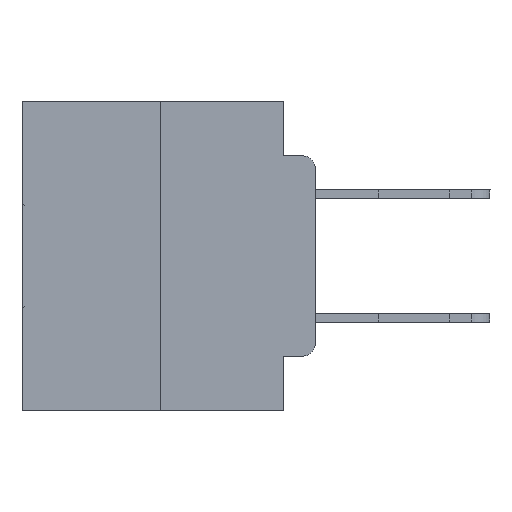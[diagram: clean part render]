
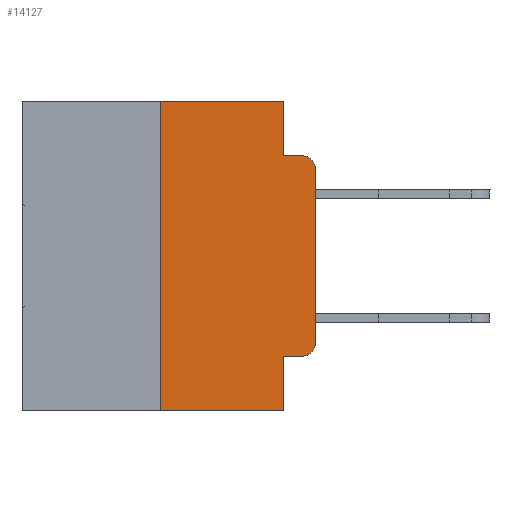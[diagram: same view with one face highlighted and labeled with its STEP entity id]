
A CAD part, left-side view. The second image highlights one B-rep face of the part: STEP entity #14127.
In plain terms, the highlighted planar face has unit normal (-1, 0, 0).
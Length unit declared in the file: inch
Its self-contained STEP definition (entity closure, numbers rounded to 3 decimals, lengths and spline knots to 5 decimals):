
#339 = VERTEX_POINT ( 'NONE', #20694 ) ;
#368 = FACE_OUTER_BOUND ( 'NONE', #4620, .T. ) ;
#550 = EDGE_CURVE ( 'NONE', #7592, #339, #29365, .T. ) ;
#661 = DIRECTION ( 'NONE',  ( 0., 0., 1. ) ) ;
#907 = VERTEX_POINT ( 'NONE', #26722 ) ;
#1243 = EDGE_CURVE ( 'NONE', #19938, #11491, #5104, .T. ) ;
#1261 = VERTEX_POINT ( 'NONE', #19348 ) ;
#1694 = CARTESIAN_POINT ( 'NONE',  ( 0., 0.25, -0.5 ) ) ;
#1778 = ORIENTED_EDGE ( 'NONE', *, *, #4622, .T. ) ;
#2238 = EDGE_CURVE ( 'NONE', #6385, #19938, #10428, .T. ) ;
#2286 = DIRECTION ( 'NONE',  ( 0., -1., 0. ) ) ;
#2720 = VERTEX_POINT ( 'NONE', #26988 ) ;
#2771 = ORIENTED_EDGE ( 'NONE', *, *, #16268, .T. ) ;
#4373 = EDGE_CURVE ( 'NONE', #11491, #29666, #7244, .T. ) ;
#4470 = DIRECTION ( 'NONE',  ( 0., 0., 1. ) ) ;
#4620 = EDGE_LOOP ( 'NONE', ( #10650, #1778, #25724, #21101, #4972, #10663, #8240, #24957, #2771, #24955 ) ) ;
#4622 = EDGE_CURVE ( 'NONE', #907, #29666, #18809, .T. ) ;
#4972 = ORIENTED_EDGE ( 'NONE', *, *, #2238, .F. ) ;
#5085 = CARTESIAN_POINT ( 'NONE',  ( 0., 0.02, -0.0885 ) ) ;
#5104 = LINE ( 'NONE', #14579, #22523 ) ;
#6385 = VERTEX_POINT ( 'NONE', #15897 ) ;
#7244 = LINE ( 'NONE', #24064, #23131 ) ;
#7370 = DIRECTION ( 'NONE',  ( 0., -1., 0. ) ) ;
#7449 = DIRECTION ( 'NONE',  ( 1., 0., 0. ) ) ;
#7592 = VERTEX_POINT ( 'NONE', #12209 ) ;
#7900 = LINE ( 'NONE', #9361, #16735 ) ;
#8240 = ORIENTED_EDGE ( 'NONE', *, *, #13862, .T. ) ;
#9361 = CARTESIAN_POINT ( 'NONE',  ( 0., 0.25, 0. ) ) ;
#9560 = VECTOR ( 'NONE', #15270, 39.37008 ) ;
#9858 = CARTESIAN_POINT ( 'NONE',  ( 0., 0.02, -0.1085 ) ) ;
#10428 = LINE ( 'NONE', #15689, #28960 ) ;
#10650 = ORIENTED_EDGE ( 'NONE', *, *, #13244, .T. ) ;
#10663 = ORIENTED_EDGE ( 'NONE', *, *, #23380, .F. ) ;
#11491 = VERTEX_POINT ( 'NONE', #19467 ) ;
#12209 = CARTESIAN_POINT ( 'NONE',  ( 0., 0.051, -0.4115 ) ) ;
#12230 = DIRECTION ( 'NONE',  ( 0., 0., -1. ) ) ;
#12478 = LINE ( 'NONE', #26468, #15379 ) ;
#13244 = EDGE_CURVE ( 'NONE', #1261, #907, #30216, .T. ) ;
#13862 = EDGE_CURVE ( 'NONE', #24104, #339, #12478, .T. ) ;
#13923 = CARTESIAN_POINT ( 'NONE',  ( 0., 0., 0. ) ) ;
#14127 = ADVANCED_FACE ( 'NONE', ( #368 ), #23072, .F. ) ;
#14579 = CARTESIAN_POINT ( 'NONE',  ( 0., 0.051, 0. ) ) ;
#15270 = DIRECTION ( 'NONE',  ( 0., 0., -1. ) ) ;
#15379 = VECTOR ( 'NONE', #7370, 39.37008 ) ;
#15689 = CARTESIAN_POINT ( 'NONE',  ( 0., 0.473, 0. ) ) ;
#15897 = CARTESIAN_POINT ( 'NONE',  ( 0., 0.25, 0. ) ) ;
#15951 = EDGE_CURVE ( 'NONE', #2720, #1261, #28708, .T. ) ;
#16268 = EDGE_CURVE ( 'NONE', #7592, #2720, #18689, .T. ) ;
#16354 = AXIS2_PLACEMENT_3D ( 'NONE', #9858, #19268, #28622 ) ;
#16735 = VECTOR ( 'NONE', #661, 39.37008 ) ;
#18030 = CARTESIAN_POINT ( 'NONE',  ( 0., 0.051, 0. ) ) ;
#18438 = VECTOR ( 'NONE', #2286, 39.37008 ) ;
#18689 = LINE ( 'NONE', #28029, #18438 ) ;
#18809 = CIRCLE ( 'NONE', #16354, 0.02 ) ;
#19268 = DIRECTION ( 'NONE',  ( -1., 0., 0. ) ) ;
#19348 = CARTESIAN_POINT ( 'NONE',  ( 0., 0., -0.3915 ) ) ;
#19373 = DIRECTION ( 'NONE',  ( 0., 0., -1. ) ) ;
#19467 = CARTESIAN_POINT ( 'NONE',  ( 0., 0.051, -0.0885 ) ) ;
#19938 = VERTEX_POINT ( 'NONE', #21917 ) ;
#20491 = DIRECTION ( 'NONE',  ( 0., 0., -1. ) ) ;
#20694 = CARTESIAN_POINT ( 'NONE',  ( 0., 0.051, -0.5 ) ) ;
#21101 = ORIENTED_EDGE ( 'NONE', *, *, #1243, .F. ) ;
#21658 = DIRECTION ( 'NONE',  ( -1., 0., 0. ) ) ;
#21917 = CARTESIAN_POINT ( 'NONE',  ( 0., 0.051, 0. ) ) ;
#22523 = VECTOR ( 'NONE', #12230, 39.37008 ) ;
#23072 = PLANE ( 'NONE',  #23215 ) ;
#23131 = VECTOR ( 'NONE', #26052, 39.37008 ) ;
#23174 = VECTOR ( 'NONE', #4470, 39.37008 ) ;
#23215 = AXIS2_PLACEMENT_3D ( 'NONE', #28562, #7449, #20491 ) ;
#23380 = EDGE_CURVE ( 'NONE', #24104, #6385, #7900, .T. ) ;
#23790 = AXIS2_PLACEMENT_3D ( 'NONE', #28573, #21658, #19373 ) ;
#24064 = CARTESIAN_POINT ( 'NONE',  ( 0., 0.051, -0.0885 ) ) ;
#24104 = VERTEX_POINT ( 'NONE', #1694 ) ;
#24955 = ORIENTED_EDGE ( 'NONE', *, *, #15951, .T. ) ;
#24957 = ORIENTED_EDGE ( 'NONE', *, *, #550, .F. ) ;
#25724 = ORIENTED_EDGE ( 'NONE', *, *, #4373, .F. ) ;
#26052 = DIRECTION ( 'NONE',  ( 0., -1., 0. ) ) ;
#26468 = CARTESIAN_POINT ( 'NONE',  ( 0., 0.473, -0.5 ) ) ;
#26722 = CARTESIAN_POINT ( 'NONE',  ( 0., 0., -0.1085 ) ) ;
#26988 = CARTESIAN_POINT ( 'NONE',  ( 0., 0.02, -0.4115 ) ) ;
#28029 = CARTESIAN_POINT ( 'NONE',  ( 0., 0.051, -0.4115 ) ) ;
#28562 = CARTESIAN_POINT ( 'NONE',  ( 0., 0.473, 0. ) ) ;
#28573 = CARTESIAN_POINT ( 'NONE',  ( 0., 0.02, -0.3915 ) ) ;
#28622 = DIRECTION ( 'NONE',  ( 0., 0., -1. ) ) ;
#28708 = CIRCLE ( 'NONE', #23790, 0.02 ) ;
#28960 = VECTOR ( 'NONE', #29333, 39.37008 ) ;
#29333 = DIRECTION ( 'NONE',  ( 0., -1., 0. ) ) ;
#29365 = LINE ( 'NONE', #18030, #9560 ) ;
#29666 = VERTEX_POINT ( 'NONE', #5085 ) ;
#30216 = LINE ( 'NONE', #13923, #23174 ) ;
